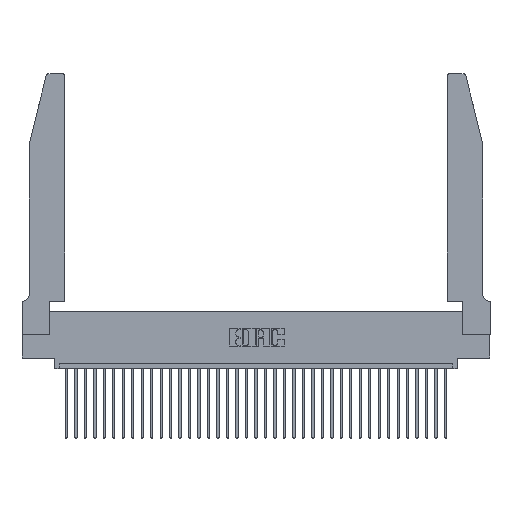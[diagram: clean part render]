
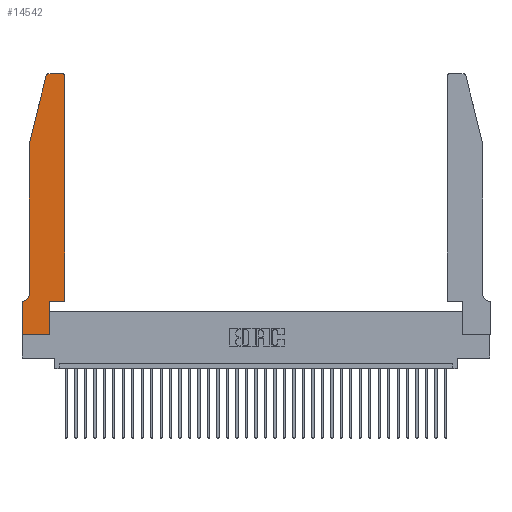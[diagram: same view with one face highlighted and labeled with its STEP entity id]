
A CAD part, top view. The second image highlights one B-rep face of the part: STEP entity #14542.
In plain terms, the highlighted planar face has unit normal (0, 0, 1).
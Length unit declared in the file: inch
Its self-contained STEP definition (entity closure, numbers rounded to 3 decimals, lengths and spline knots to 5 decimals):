
#1331 = CARTESIAN_POINT ( 'NONE',  ( 0.2865, 0.35, 0.37 ) ) ;
#2126 = LINE ( 'NONE', #7384, #30756 ) ;
#2314 = VERTEX_POINT ( 'NONE', #32561 ) ;
#2357 = DIRECTION ( 'NONE',  ( 0., -1., 0. ) ) ;
#2606 = LINE ( 'NONE', #15047, #31224 ) ;
#2844 = VECTOR ( 'NONE', #2357, 39.37008 ) ;
#2961 = CARTESIAN_POINT ( 'NONE',  ( 0., 0., 0.37 ) ) ;
#3115 = LINE ( 'NONE', #33413, #28678 ) ;
#3257 = DIRECTION ( 'NONE',  ( 1., 0., 0. ) ) ;
#3328 = CIRCLE ( 'NONE', #26267, 0.07 ) ;
#3395 = EDGE_CURVE ( 'NONE', #22340, #32439, #32327, .T. ) ;
#3563 = EDGE_CURVE ( 'NONE', #32439, #28702, #15372, .T. ) ;
#3824 = VECTOR ( 'NONE', #12013, 39.37008 ) ;
#3945 = CARTESIAN_POINT ( 'NONE',  ( 0.2865, 0., 0.37 ) ) ;
#3955 = VERTEX_POINT ( 'NONE', #11714 ) ;
#4319 = CARTESIAN_POINT ( 'NONE',  ( 0.284, 2.75, 0.37 ) ) ;
#4513 = CARTESIAN_POINT ( 'NONE',  ( 0., 0., 0.37 ) ) ;
#6264 = DIRECTION ( 'NONE',  ( 1., 0., 0. ) ) ;
#6589 = AXIS2_PLACEMENT_3D ( 'NONE', #23722, #7885, #15471 ) ;
#7353 = EDGE_CURVE ( 'NONE', #10406, #17331, #35028, .T. ) ;
#7384 = CARTESIAN_POINT ( 'NONE',  ( 0.0755, 2., 0.37 ) ) ;
#7885 = DIRECTION ( 'NONE',  ( 0., 0., 1. ) ) ;
#8003 = DIRECTION ( 'NONE',  ( 0., 0., -1. ) ) ;
#8807 = ORIENTED_EDGE ( 'NONE', *, *, #32968, .T. ) ;
#10406 = VERTEX_POINT ( 'NONE', #32893 ) ;
#11587 = VERTEX_POINT ( 'NONE', #15555 ) ;
#11714 = CARTESIAN_POINT ( 'NONE',  ( 0.0755, 2., 0.37 ) ) ;
#12013 = DIRECTION ( 'NONE',  ( -1., 0., 0. ) ) ;
#12300 = EDGE_CURVE ( 'NONE', #35132, #3955, #2126, .T. ) ;
#12601 = VERTEX_POINT ( 'NONE', #20661 ) ;
#13278 = LINE ( 'NONE', #1331, #25446 ) ;
#13910 = EDGE_CURVE ( 'NONE', #11587, #26570, #3328, .T. ) ;
#13942 = AXIS2_PLACEMENT_3D ( 'NONE', #17046, #31112, #3257 ) ;
#14265 = PLANE ( 'NONE',  #13942 ) ;
#14542 = ADVANCED_FACE ( 'NONE', ( #15806 ), #14265, .T. ) ;
#14870 = CARTESIAN_POINT ( 'NONE',  ( 0.25487, 2.72718, 0.37 ) ) ;
#15047 = CARTESIAN_POINT ( 'NONE',  ( 0.4505, 0.35, 0.37 ) ) ;
#15372 = LINE ( 'NONE', #2961, #34035 ) ;
#15394 = DIRECTION ( 'NONE',  ( 0., 1., 0. ) ) ;
#15438 = DIRECTION ( 'NONE',  ( 1., 0., 0. ) ) ;
#15471 = DIRECTION ( 'NONE',  ( 1., 0., 0. ) ) ;
#15555 = CARTESIAN_POINT ( 'NONE',  ( 0.0755, 0.42, 0.37 ) ) ;
#15614 = ORIENTED_EDGE ( 'NONE', *, *, #12300, .T. ) ;
#15626 = EDGE_LOOP ( 'NONE', ( #18121, #20255, #15614, #31020, #27216, #22582, #20705, #29442, #8807, #16844, #17479, #18748 ) ) ;
#15806 = FACE_OUTER_BOUND ( 'NONE', #15626, .T. ) ;
#15935 = EDGE_CURVE ( 'NONE', #17331, #35132, #34244, .T. ) ;
#16553 = EDGE_CURVE ( 'NONE', #18317, #12601, #19952, .T. ) ;
#16844 = ORIENTED_EDGE ( 'NONE', *, *, #16553, .T. ) ;
#16914 = DIRECTION ( 'NONE',  ( -1., 0., 0. ) ) ;
#17046 = CARTESIAN_POINT ( 'NONE',  ( 0., 0.35, 0.37 ) ) ;
#17105 = CARTESIAN_POINT ( 'NONE',  ( 0.2865, 0.35, 0.37 ) ) ;
#17331 = VERTEX_POINT ( 'NONE', #4319 ) ;
#17479 = ORIENTED_EDGE ( 'NONE', *, *, #24621, .T. ) ;
#18121 = ORIENTED_EDGE ( 'NONE', *, *, #7353, .T. ) ;
#18317 = VERTEX_POINT ( 'NONE', #17105 ) ;
#18748 = ORIENTED_EDGE ( 'NONE', *, *, #22366, .T. ) ;
#19952 = LINE ( 'NONE', #31717, #28615 ) ;
#20255 = ORIENTED_EDGE ( 'NONE', *, *, #15935, .T. ) ;
#20661 = CARTESIAN_POINT ( 'NONE',  ( 0.4505, 0.35, 0.37 ) ) ;
#20705 = ORIENTED_EDGE ( 'NONE', *, *, #3395, .T. ) ;
#20712 = DIRECTION ( 'NONE',  ( 0., 1., 0. ) ) ;
#20873 = EDGE_CURVE ( 'NONE', #3955, #11587, #30861, .T. ) ;
#22210 = VECTOR ( 'NONE', #25806, 39.37008 ) ;
#22238 = CARTESIAN_POINT ( 'NONE',  ( 0., 0., 0.37 ) ) ;
#22340 = VERTEX_POINT ( 'NONE', #22385 ) ;
#22366 = EDGE_CURVE ( 'NONE', #2314, #10406, #30068, .T. ) ;
#22385 = CARTESIAN_POINT ( 'NONE',  ( 0., 0.35, 0.37 ) ) ;
#22582 = ORIENTED_EDGE ( 'NONE', *, *, #35572, .T. ) ;
#23722 = CARTESIAN_POINT ( 'NONE',  ( 0.284, 2.72, 0.37 ) ) ;
#24342 = CARTESIAN_POINT ( 'NONE',  ( 0.0055, 0.35, 0.37 ) ) ;
#24621 = EDGE_CURVE ( 'NONE', #12601, #2314, #2606, .T. ) ;
#25388 = DIRECTION ( 'NONE',  ( 1., 0., 0. ) ) ;
#25446 = VECTOR ( 'NONE', #20712, 39.37008 ) ;
#25806 = DIRECTION ( 'NONE',  ( 0., -1., 0. ) ) ;
#26267 = AXIS2_PLACEMENT_3D ( 'NONE', #35606, #8003, #28173 ) ;
#26570 = VERTEX_POINT ( 'NONE', #24342 ) ;
#27216 = ORIENTED_EDGE ( 'NONE', *, *, #13910, .T. ) ;
#28173 = DIRECTION ( 'NONE',  ( -1., 0., 0. ) ) ;
#28604 = CARTESIAN_POINT ( 'NONE',  ( 0.2605, 2.75, 0.37 ) ) ;
#28615 = VECTOR ( 'NONE', #15438, 39.37008 ) ;
#28678 = VECTOR ( 'NONE', #16914, 39.37008 ) ;
#28702 = VERTEX_POINT ( 'NONE', #3945 ) ;
#29442 = ORIENTED_EDGE ( 'NONE', *, *, #3563, .T. ) ;
#29453 = AXIS2_PLACEMENT_3D ( 'NONE', #34229, #31572, #6264 ) ;
#30068 = CIRCLE ( 'NONE', #29453, 0.03 ) ;
#30756 = VECTOR ( 'NONE', #32710, 39.37008 ) ;
#30784 = CARTESIAN_POINT ( 'NONE',  ( 0.0755, 2., 0.37 ) ) ;
#30861 = LINE ( 'NONE', #30784, #22210 ) ;
#31020 = ORIENTED_EDGE ( 'NONE', *, *, #20873, .T. ) ;
#31112 = DIRECTION ( 'NONE',  ( 0., 0., 1. ) ) ;
#31224 = VECTOR ( 'NONE', #15394, 39.37008 ) ;
#31572 = DIRECTION ( 'NONE',  ( 0., 0., 1. ) ) ;
#31717 = CARTESIAN_POINT ( 'NONE',  ( 0.4505, 0.35, 0.37 ) ) ;
#32327 = LINE ( 'NONE', #22238, #2844 ) ;
#32439 = VERTEX_POINT ( 'NONE', #4513 ) ;
#32561 = CARTESIAN_POINT ( 'NONE',  ( 0.4505, 2.72, 0.37 ) ) ;
#32710 = DIRECTION ( 'NONE',  ( -0.239, -0.971, 0. ) ) ;
#32893 = CARTESIAN_POINT ( 'NONE',  ( 0.4205, 2.75, 0.37 ) ) ;
#32968 = EDGE_CURVE ( 'NONE', #28702, #18317, #13278, .T. ) ;
#33413 = CARTESIAN_POINT ( 'NONE',  ( 0.0755, 0.35, 0.37 ) ) ;
#34035 = VECTOR ( 'NONE', #25388, 39.37008 ) ;
#34229 = CARTESIAN_POINT ( 'NONE',  ( 0.4205, 2.72, 0.37 ) ) ;
#34244 = CIRCLE ( 'NONE', #6589, 0.03 ) ;
#35028 = LINE ( 'NONE', #28604, #3824 ) ;
#35132 = VERTEX_POINT ( 'NONE', #14870 ) ;
#35572 = EDGE_CURVE ( 'NONE', #26570, #22340, #3115, .T. ) ;
#35606 = CARTESIAN_POINT ( 'NONE',  ( 0.0055, 0.42, 0.37 ) ) ;
